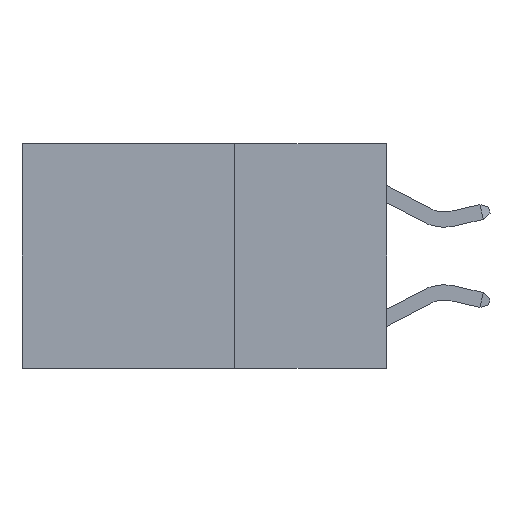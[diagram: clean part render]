
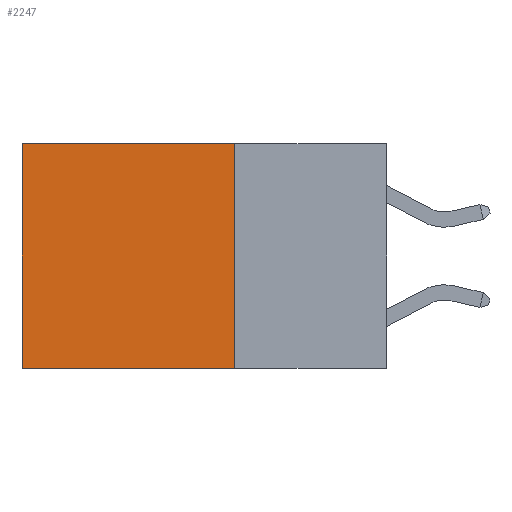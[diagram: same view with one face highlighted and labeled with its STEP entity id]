
A CAD part, left-side view. The second image highlights one B-rep face of the part: STEP entity #2247.
In plain terms, the highlighted planar face has unit normal (-1, 0, 0).
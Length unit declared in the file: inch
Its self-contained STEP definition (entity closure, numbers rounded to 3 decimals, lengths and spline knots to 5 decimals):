
#62 = EDGE_CURVE ( 'NONE', #5326, #7328, #982, .T. ) ;
#625 = DIRECTION ( 'NONE',  ( 0., 0., -1. ) ) ;
#733 = DIRECTION ( 'NONE',  ( 0., 1., 0. ) ) ;
#982 = LINE ( 'NONE', #8603, #4479 ) ;
#986 = DIRECTION ( 'NONE',  ( 1., 0., 0. ) ) ;
#1535 = CARTESIAN_POINT ( 'NONE',  ( 0.2625, 0.25, 0. ) ) ;
#1572 = CARTESIAN_POINT ( 'NONE',  ( 0.2625, 0.6, -0.37 ) ) ;
#2059 = CARTESIAN_POINT ( 'NONE',  ( 0.2625, 0.25, 0. ) ) ;
#2247 = ADVANCED_FACE ( 'NONE', ( #4328 ), #3152, .F. ) ;
#2421 = LINE ( 'NONE', #2059, #2639 ) ;
#2458 = VERTEX_POINT ( 'NONE', #2713 ) ;
#2639 = VECTOR ( 'NONE', #625, 39.37008 ) ;
#2713 = CARTESIAN_POINT ( 'NONE',  ( 0.2625, 0.6, 0. ) ) ;
#2922 = DIRECTION ( 'NONE',  ( 0., 0., -1. ) ) ;
#2954 = EDGE_CURVE ( 'NONE', #2458, #7328, #7913, .T. ) ;
#3019 = ORIENTED_EDGE ( 'NONE', *, *, #62, .F. ) ;
#3135 = VECTOR ( 'NONE', #8397, 39.37008 ) ;
#3152 = PLANE ( 'NONE',  #8310 ) ;
#3366 = EDGE_LOOP ( 'NONE', ( #4937, #3019, #4939, #4791 ) ) ;
#4238 = CARTESIAN_POINT ( 'NONE',  ( 0.2625, 0.25, -0.37 ) ) ;
#4313 = VECTOR ( 'NONE', #4943, 39.37008 ) ;
#4328 = FACE_OUTER_BOUND ( 'NONE', #3366, .T. ) ;
#4479 = VECTOR ( 'NONE', #733, 39.37008 ) ;
#4668 = VERTEX_POINT ( 'NONE', #1535 ) ;
#4791 = ORIENTED_EDGE ( 'NONE', *, *, #7978, .T. ) ;
#4937 = ORIENTED_EDGE ( 'NONE', *, *, #2954, .T. ) ;
#4939 = ORIENTED_EDGE ( 'NONE', *, *, #5257, .F. ) ;
#4943 = DIRECTION ( 'NONE',  ( 0., 0., -1. ) ) ;
#4987 = CARTESIAN_POINT ( 'NONE',  ( 0.2625, 0.6, 0. ) ) ;
#5257 = EDGE_CURVE ( 'NONE', #4668, #5326, #2421, .T. ) ;
#5326 = VERTEX_POINT ( 'NONE', #4238 ) ;
#6021 = CARTESIAN_POINT ( 'NONE',  ( 0.2625, 0.25, 0. ) ) ;
#6756 = LINE ( 'NONE', #7692, #3135 ) ;
#7328 = VERTEX_POINT ( 'NONE', #1572 ) ;
#7692 = CARTESIAN_POINT ( 'NONE',  ( 0.2625, 0.25, 0. ) ) ;
#7913 = LINE ( 'NONE', #4987, #4313 ) ;
#7978 = EDGE_CURVE ( 'NONE', #4668, #2458, #6756, .T. ) ;
#8310 = AXIS2_PLACEMENT_3D ( 'NONE', #6021, #986, #2922 ) ;
#8397 = DIRECTION ( 'NONE',  ( 0., 1., 0. ) ) ;
#8603 = CARTESIAN_POINT ( 'NONE',  ( 0.2625, 0.25, -0.37 ) ) ;
